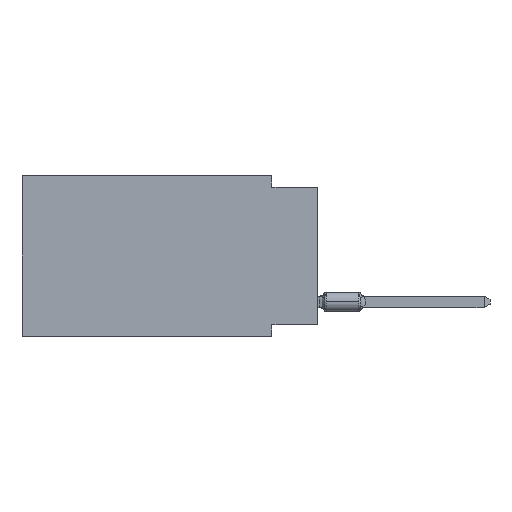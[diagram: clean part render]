
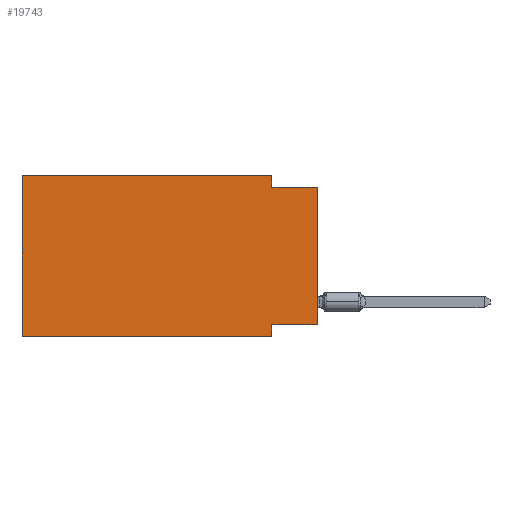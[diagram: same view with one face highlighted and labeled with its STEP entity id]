
A CAD part, left-side view. The second image highlights one B-rep face of the part: STEP entity #19743.
In plain terms, the highlighted planar face has unit normal (-1, 0, 0).
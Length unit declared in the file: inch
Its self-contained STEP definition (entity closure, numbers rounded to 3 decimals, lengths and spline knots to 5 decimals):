
#47 = CARTESIAN_POINT ( 'NONE',  ( 0., 0., -0.025 ) ) ;
#716 = EDGE_CURVE ( 'NONE', #1627, #3820, #919, .T. ) ;
#919 = LINE ( 'NONE', #28125, #21762 ) ;
#1625 = CARTESIAN_POINT ( 'NONE',  ( 0., 0.1, 0. ) ) ;
#1627 = VERTEX_POINT ( 'NONE', #14751 ) ;
#2583 = EDGE_CURVE ( 'NONE', #24337, #1627, #25372, .T. ) ;
#2695 = DIRECTION ( 'NONE',  ( 0., 0., 1. ) ) ;
#2765 = VECTOR ( 'NONE', #7101, 39.37008 ) ;
#2839 = CARTESIAN_POINT ( 'NONE',  ( 0., 0.645, 0. ) ) ;
#3751 = VECTOR ( 'NONE', #17346, 39.37008 ) ;
#3820 = VERTEX_POINT ( 'NONE', #16411 ) ;
#4118 = VECTOR ( 'NONE', #10254, 39.37008 ) ;
#4785 = ORIENTED_EDGE ( 'NONE', *, *, #5829, .F. ) ;
#5000 = ORIENTED_EDGE ( 'NONE', *, *, #716, .F. ) ;
#5468 = EDGE_CURVE ( 'NONE', #24337, #8626, #18088, .T. ) ;
#5541 = ORIENTED_EDGE ( 'NONE', *, *, #7493, .T. ) ;
#5829 = EDGE_CURVE ( 'NONE', #12566, #8626, #20101, .T. ) ;
#5877 = CARTESIAN_POINT ( 'NONE',  ( 0., 0., -0.325 ) ) ;
#6344 = DIRECTION ( 'NONE',  ( 0., 0., -1. ) ) ;
#6917 = VECTOR ( 'NONE', #11921, 39.37008 ) ;
#6966 = CARTESIAN_POINT ( 'NONE',  ( 0., 0.645, -0.35 ) ) ;
#7101 = DIRECTION ( 'NONE',  ( 0., -1., 0. ) ) ;
#7493 = EDGE_CURVE ( 'NONE', #24992, #25685, #18363, .T. ) ;
#8626 = VERTEX_POINT ( 'NONE', #27726 ) ;
#8675 = FACE_OUTER_BOUND ( 'NONE', #25281, .T. ) ;
#8823 = ORIENTED_EDGE ( 'NONE', *, *, #18844, .F. ) ;
#9750 = CARTESIAN_POINT ( 'NONE',  ( 0., 0.1, -0.025 ) ) ;
#9958 = ORIENTED_EDGE ( 'NONE', *, *, #5468, .T. ) ;
#10004 = CARTESIAN_POINT ( 'NONE',  ( 0., 0.1, -0.325 ) ) ;
#10122 = EDGE_CURVE ( 'NONE', #24992, #12566, #16854, .T. ) ;
#10254 = DIRECTION ( 'NONE',  ( 0., 0., -1. ) ) ;
#10745 = VECTOR ( 'NONE', #2695, 39.37008 ) ;
#10997 = EDGE_CURVE ( 'NONE', #20783, #25685, #26679, .T. ) ;
#11921 = DIRECTION ( 'NONE',  ( 0., 0., 1. ) ) ;
#12144 = ORIENTED_EDGE ( 'NONE', *, *, #10997, .F. ) ;
#12566 = VERTEX_POINT ( 'NONE', #10004 ) ;
#12733 = DIRECTION ( 'NONE',  ( 0., 1., 0. ) ) ;
#12979 = VECTOR ( 'NONE', #24493, 39.37008 ) ;
#14751 = CARTESIAN_POINT ( 'NONE',  ( 0., 0.645, 0. ) ) ;
#16411 = CARTESIAN_POINT ( 'NONE',  ( 0., 0.1, 0. ) ) ;
#16689 = ORIENTED_EDGE ( 'NONE', *, *, #2583, .F. ) ;
#16854 = LINE ( 'NONE', #5877, #17619 ) ;
#17346 = DIRECTION ( 'NONE',  ( 0., 0., -1. ) ) ;
#17352 = CARTESIAN_POINT ( 'NONE',  ( 0., 0., -0.025 ) ) ;
#17610 = PLANE ( 'NONE',  #19071 ) ;
#17619 = VECTOR ( 'NONE', #12733, 39.37008 ) ;
#18088 = LINE ( 'NONE', #6966, #2765 ) ;
#18363 = LINE ( 'NONE', #23043, #6917 ) ;
#18844 = EDGE_CURVE ( 'NONE', #3820, #20783, #25911, .T. ) ;
#19071 = AXIS2_PLACEMENT_3D ( 'NONE', #24336, #26396, #6344 ) ;
#19743 = ADVANCED_FACE ( 'NONE', ( #8675 ), #17610, .F. ) ;
#20101 = LINE ( 'NONE', #28473, #3751 ) ;
#20783 = VERTEX_POINT ( 'NONE', #9750 ) ;
#21245 = DIRECTION ( 'NONE',  ( 0., -1., 0. ) ) ;
#21762 = VECTOR ( 'NONE', #21245, 39.37008 ) ;
#22180 = ORIENTED_EDGE ( 'NONE', *, *, #10122, .F. ) ;
#22955 = CARTESIAN_POINT ( 'NONE',  ( 0., 0., -0.325 ) ) ;
#23043 = CARTESIAN_POINT ( 'NONE',  ( 0., 0., 0. ) ) ;
#24336 = CARTESIAN_POINT ( 'NONE',  ( 0., 0.645, 0. ) ) ;
#24337 = VERTEX_POINT ( 'NONE', #26534 ) ;
#24493 = DIRECTION ( 'NONE',  ( 0., -1., 0. ) ) ;
#24992 = VERTEX_POINT ( 'NONE', #22955 ) ;
#25281 = EDGE_LOOP ( 'NONE', ( #5541, #12144, #8823, #5000, #16689, #9958, #4785, #22180 ) ) ;
#25372 = LINE ( 'NONE', #2839, #10745 ) ;
#25685 = VERTEX_POINT ( 'NONE', #17352 ) ;
#25911 = LINE ( 'NONE', #1625, #4118 ) ;
#26396 = DIRECTION ( 'NONE',  ( 1., 0., 0. ) ) ;
#26534 = CARTESIAN_POINT ( 'NONE',  ( 0., 0.645, -0.35 ) ) ;
#26679 = LINE ( 'NONE', #47, #12979 ) ;
#27726 = CARTESIAN_POINT ( 'NONE',  ( 0., 0.1, -0.35 ) ) ;
#28125 = CARTESIAN_POINT ( 'NONE',  ( 0., 0.645, 0. ) ) ;
#28473 = CARTESIAN_POINT ( 'NONE',  ( 0., 0.1, -0.35 ) ) ;
